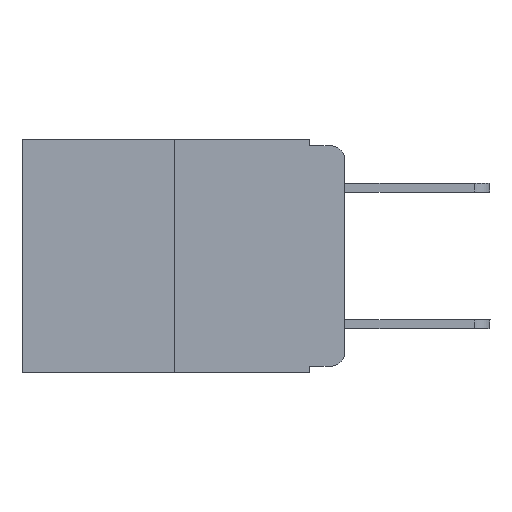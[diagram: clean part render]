
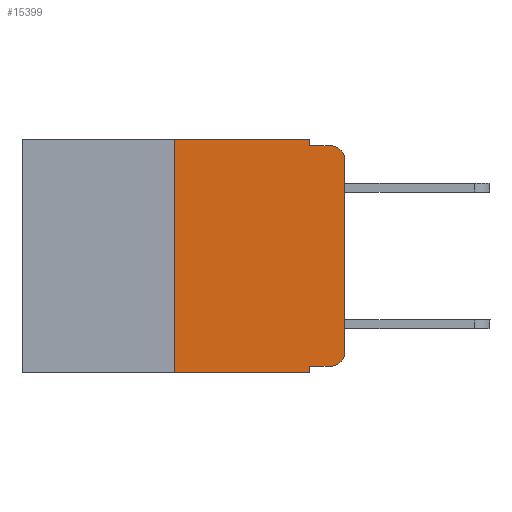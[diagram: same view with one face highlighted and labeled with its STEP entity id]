
A CAD part, left-side view. The second image highlights one B-rep face of the part: STEP entity #15399.
In plain terms, the highlighted planar face has unit normal (-1, 0, 0).
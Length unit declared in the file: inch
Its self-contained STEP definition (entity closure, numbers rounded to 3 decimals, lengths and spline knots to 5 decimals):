
#29 = DIRECTION ( 'NONE',  ( 0., 0., 1. ) ) ;
#37 = VERTEX_POINT ( 'NONE', #15624 ) ;
#122 = LINE ( 'NONE', #11393, #4287 ) ;
#1374 = CARTESIAN_POINT ( 'NONE',  ( 0., 0.051, -0.343 ) ) ;
#1427 = CARTESIAN_POINT ( 'NONE',  ( 0., 0.25, 0. ) ) ;
#1799 = DIRECTION ( 'NONE',  ( 0., -1., 0. ) ) ;
#1894 = CARTESIAN_POINT ( 'NONE',  ( 0., 0.02, -0.333 ) ) ;
#1897 = CARTESIAN_POINT ( 'NONE',  ( 0., 0., -0.313 ) ) ;
#2097 = CARTESIAN_POINT ( 'NONE',  ( 0., 0.02, -0.03 ) ) ;
#2241 = LINE ( 'NONE', #14880, #10535 ) ;
#2839 = CARTESIAN_POINT ( 'NONE',  ( 0., 0.25, 0. ) ) ;
#3163 = DIRECTION ( 'NONE',  ( -1., 0., 0. ) ) ;
#3307 = ORIENTED_EDGE ( 'NONE', *, *, #8018, .F. ) ;
#3341 = CARTESIAN_POINT ( 'NONE',  ( 0., 0.473, 0. ) ) ;
#3450 = PLANE ( 'NONE',  #10299 ) ;
#3624 = VECTOR ( 'NONE', #15207, 39.37008 ) ;
#4015 = VERTEX_POINT ( 'NONE', #1374 ) ;
#4058 = DIRECTION ( 'NONE',  ( 0., 0., 1. ) ) ;
#4287 = VECTOR ( 'NONE', #1799, 39.37008 ) ;
#4559 = DIRECTION ( 'NONE',  ( 0., -1., 0. ) ) ;
#4747 = DIRECTION ( 'NONE',  ( 0., -1., 0. ) ) ;
#4765 = DIRECTION ( 'NONE',  ( 0., 0., -1. ) ) ;
#4823 = DIRECTION ( 'NONE',  ( 0., 0., -1. ) ) ;
#5008 = LINE ( 'NONE', #10384, #15116 ) ;
#5257 = LINE ( 'NONE', #8690, #10734 ) ;
#5386 = VERTEX_POINT ( 'NONE', #1894 ) ;
#5401 = EDGE_CURVE ( 'NONE', #12018, #8128, #5257, .T. ) ;
#5569 = CARTESIAN_POINT ( 'NONE',  ( 0., 0.051, 0. ) ) ;
#5732 = VERTEX_POINT ( 'NONE', #15185 ) ;
#5774 = AXIS2_PLACEMENT_3D ( 'NONE', #2097, #11641, #4823 ) ;
#5888 = CARTESIAN_POINT ( 'NONE',  ( 0., 0.473, -0.343 ) ) ;
#6242 = CIRCLE ( 'NONE', #5774, 0.02 ) ;
#6333 = CARTESIAN_POINT ( 'NONE',  ( 0., 0.051, -0.333 ) ) ;
#6842 = VERTEX_POINT ( 'NONE', #1897 ) ;
#7413 = DIRECTION ( 'NONE',  ( 0., 0., -1. ) ) ;
#8018 = EDGE_CURVE ( 'NONE', #37, #15819, #15082, .T. ) ;
#8128 = VERTEX_POINT ( 'NONE', #10510 ) ;
#8690 = CARTESIAN_POINT ( 'NONE',  ( 0., 0.051, -0.01 ) ) ;
#8842 = ORIENTED_EDGE ( 'NONE', *, *, #11287, .F. ) ;
#8972 = EDGE_CURVE ( 'NONE', #17915, #5386, #122, .T. ) ;
#9008 = LINE ( 'NONE', #5888, #16935 ) ;
#9041 = EDGE_CURVE ( 'NONE', #5386, #6842, #10408, .T. ) ;
#9073 = EDGE_CURVE ( 'NONE', #5732, #8128, #6242, .T. ) ;
#9545 = ORIENTED_EDGE ( 'NONE', *, *, #12975, .T. ) ;
#9725 = CARTESIAN_POINT ( 'NONE',  ( 0., 0., 0. ) ) ;
#10120 = EDGE_CURVE ( 'NONE', #6842, #5732, #10585, .T. ) ;
#10299 = AXIS2_PLACEMENT_3D ( 'NONE', #3341, #14553, #4765 ) ;
#10384 = CARTESIAN_POINT ( 'NONE',  ( 0., 0.473, 0. ) ) ;
#10408 = CIRCLE ( 'NONE', #11511, 0.02 ) ;
#10510 = CARTESIAN_POINT ( 'NONE',  ( 0., 0.02, -0.01 ) ) ;
#10535 = VECTOR ( 'NONE', #16289, 39.37008 ) ;
#10585 = LINE ( 'NONE', #9725, #16757 ) ;
#10722 = ORIENTED_EDGE ( 'NONE', *, *, #5401, .F. ) ;
#10734 = VECTOR ( 'NONE', #4559, 39.37008 ) ;
#10758 = ORIENTED_EDGE ( 'NONE', *, *, #16167, .F. ) ;
#11287 = EDGE_CURVE ( 'NONE', #17915, #4015, #2241, .T. ) ;
#11393 = CARTESIAN_POINT ( 'NONE',  ( 0., 0.051, -0.333 ) ) ;
#11511 = AXIS2_PLACEMENT_3D ( 'NONE', #17118, #3163, #7413 ) ;
#11641 = DIRECTION ( 'NONE',  ( -1., 0., 0. ) ) ;
#11657 = DIRECTION ( 'NONE',  ( 0., -1., 0. ) ) ;
#12018 = VERTEX_POINT ( 'NONE', #13811 ) ;
#12975 = EDGE_CURVE ( 'NONE', #37, #4015, #9008, .T. ) ;
#13671 = CARTESIAN_POINT ( 'NONE',  ( 0., 0.051, 0. ) ) ;
#13811 = CARTESIAN_POINT ( 'NONE',  ( 0., 0.051, -0.01 ) ) ;
#14124 = EDGE_CURVE ( 'NONE', #15819, #15764, #5008, .T. ) ;
#14265 = EDGE_LOOP ( 'NONE', ( #14532, #15551, #10722, #10758, #17709, #3307, #9545, #8842, #16902, #14678 ) ) ;
#14532 = ORIENTED_EDGE ( 'NONE', *, *, #10120, .T. ) ;
#14553 = DIRECTION ( 'NONE',  ( 1., 0., 0. ) ) ;
#14678 = ORIENTED_EDGE ( 'NONE', *, *, #9041, .T. ) ;
#14813 = LINE ( 'NONE', #13671, #3624 ) ;
#14880 = CARTESIAN_POINT ( 'NONE',  ( 0., 0.051, 0. ) ) ;
#15082 = LINE ( 'NONE', #1427, #15306 ) ;
#15116 = VECTOR ( 'NONE', #4747, 39.37008 ) ;
#15185 = CARTESIAN_POINT ( 'NONE',  ( 0., 0., -0.03 ) ) ;
#15207 = DIRECTION ( 'NONE',  ( 0., 0., -1. ) ) ;
#15306 = VECTOR ( 'NONE', #4058, 39.37008 ) ;
#15399 = ADVANCED_FACE ( 'NONE', ( #16151 ), #3450, .F. ) ;
#15551 = ORIENTED_EDGE ( 'NONE', *, *, #9073, .T. ) ;
#15624 = CARTESIAN_POINT ( 'NONE',  ( 0., 0.25, -0.343 ) ) ;
#15764 = VERTEX_POINT ( 'NONE', #5569 ) ;
#15819 = VERTEX_POINT ( 'NONE', #2839 ) ;
#16151 = FACE_OUTER_BOUND ( 'NONE', #14265, .T. ) ;
#16167 = EDGE_CURVE ( 'NONE', #15764, #12018, #14813, .T. ) ;
#16289 = DIRECTION ( 'NONE',  ( 0., 0., -1. ) ) ;
#16757 = VECTOR ( 'NONE', #29, 39.37008 ) ;
#16902 = ORIENTED_EDGE ( 'NONE', *, *, #8972, .T. ) ;
#16935 = VECTOR ( 'NONE', #11657, 39.37008 ) ;
#17118 = CARTESIAN_POINT ( 'NONE',  ( 0., 0.02, -0.313 ) ) ;
#17709 = ORIENTED_EDGE ( 'NONE', *, *, #14124, .F. ) ;
#17915 = VERTEX_POINT ( 'NONE', #6333 ) ;
